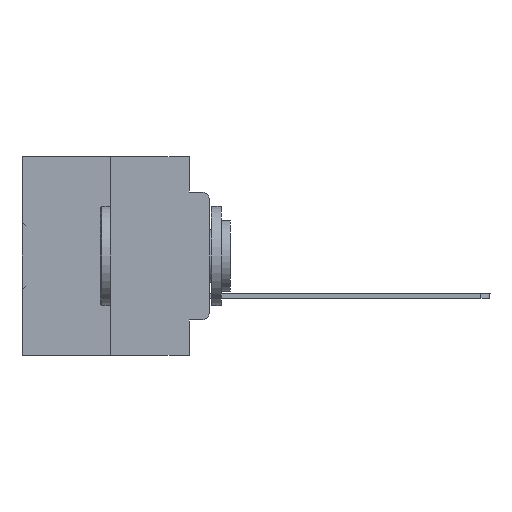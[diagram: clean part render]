
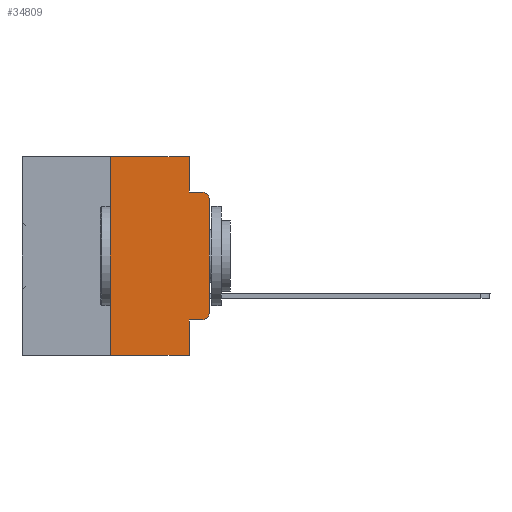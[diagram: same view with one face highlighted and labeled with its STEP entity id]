
A CAD part, left-side view. The second image highlights one B-rep face of the part: STEP entity #34809.
In plain terms, the highlighted planar face has unit normal (-1, 0, 0).
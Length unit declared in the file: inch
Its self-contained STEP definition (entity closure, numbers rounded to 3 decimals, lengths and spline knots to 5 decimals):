
#565 = VECTOR ( 'NONE', #27061, 39.37008 ) ;
#676 = CARTESIAN_POINT ( 'NONE',  ( 0., 0.051, -0.0885 ) ) ;
#716 = DIRECTION ( 'NONE',  ( -1., 0., 0. ) ) ;
#834 = CARTESIAN_POINT ( 'NONE',  ( 0., 0.051, -0.4115 ) ) ;
#895 = ORIENTED_EDGE ( 'NONE', *, *, #23090, .T. ) ;
#981 = LINE ( 'NONE', #23210, #13466 ) ;
#1661 = DIRECTION ( 'NONE',  ( 0., -1., 0. ) ) ;
#2982 = EDGE_CURVE ( 'NONE', #19522, #21882, #26167, .T. ) ;
#3348 = CARTESIAN_POINT ( 'NONE',  ( 0., 0.473, 0. ) ) ;
#4129 = CARTESIAN_POINT ( 'NONE',  ( 0., 0.473, -0.5 ) ) ;
#4515 = EDGE_CURVE ( 'NONE', #19522, #31676, #13533, .T. ) ;
#4795 = CARTESIAN_POINT ( 'NONE',  ( 0., 0., 0. ) ) ;
#4839 = VERTEX_POINT ( 'NONE', #7414 ) ;
#6192 = VECTOR ( 'NONE', #35903, 39.37008 ) ;
#6495 = EDGE_CURVE ( 'NONE', #4839, #33260, #25482, .T. ) ;
#6571 = ORIENTED_EDGE ( 'NONE', *, *, #23447, .T. ) ;
#7414 = CARTESIAN_POINT ( 'NONE',  ( 0., 0.25, -0.5 ) ) ;
#7558 = LINE ( 'NONE', #18197, #15893 ) ;
#7573 = VECTOR ( 'NONE', #21011, 39.37008 ) ;
#9270 = EDGE_CURVE ( 'NONE', #21882, #29329, #12738, .T. ) ;
#9669 = CARTESIAN_POINT ( 'NONE',  ( 0., 0., -0.3915 ) ) ;
#10078 = VECTOR ( 'NONE', #34612, 39.37008 ) ;
#10139 = LINE ( 'NONE', #4795, #32683 ) ;
#10311 = EDGE_LOOP ( 'NONE', ( #6571, #895, #25786, #10936, #17697, #33186, #24774, #27857, #26326, #21226 ) ) ;
#10936 = ORIENTED_EDGE ( 'NONE', *, *, #33438, .F. ) ;
#11402 = EDGE_CURVE ( 'NONE', #16914, #16169, #12222, .T. ) ;
#12222 = LINE ( 'NONE', #18078, #7573 ) ;
#12738 = CIRCLE ( 'NONE', #29735, 0.02 ) ;
#13162 = CARTESIAN_POINT ( 'NONE',  ( 0., 0.051, -0.4115 ) ) ;
#13466 = VECTOR ( 'NONE', #25590, 39.37008 ) ;
#13533 = LINE ( 'NONE', #24704, #6192 ) ;
#13666 = CARTESIAN_POINT ( 'NONE',  ( 0., 0.02, -0.1085 ) ) ;
#13837 = DIRECTION ( 'NONE',  ( 0., 0., -1. ) ) ;
#14575 = DIRECTION ( 'NONE',  ( 1., 0., 0. ) ) ;
#15657 = CARTESIAN_POINT ( 'NONE',  ( 0., 0.02, -0.0885 ) ) ;
#15854 = EDGE_CURVE ( 'NONE', #4839, #31676, #16072, .T. ) ;
#15893 = VECTOR ( 'NONE', #1661, 39.37008 ) ;
#16072 = LINE ( 'NONE', #4129, #565 ) ;
#16169 = VERTEX_POINT ( 'NONE', #15657 ) ;
#16354 = VECTOR ( 'NONE', #28792, 39.37008 ) ;
#16914 = VERTEX_POINT ( 'NONE', #676 ) ;
#17449 = AXIS2_PLACEMENT_3D ( 'NONE', #13666, #22075, #13837 ) ;
#17697 = ORIENTED_EDGE ( 'NONE', *, *, #28563, .F. ) ;
#18078 = CARTESIAN_POINT ( 'NONE',  ( 0., 0.051, -0.0885 ) ) ;
#18197 = CARTESIAN_POINT ( 'NONE',  ( 0., 0.473, 0. ) ) ;
#18350 = CARTESIAN_POINT ( 'NONE',  ( 0., 0.02, -0.3915 ) ) ;
#18533 = CARTESIAN_POINT ( 'NONE',  ( 0., 0., -0.1085 ) ) ;
#19384 = CARTESIAN_POINT ( 'NONE',  ( 0., 0.25, 0. ) ) ;
#19522 = VERTEX_POINT ( 'NONE', #13162 ) ;
#20610 = DIRECTION ( 'NONE',  ( 0., 0., -1. ) ) ;
#21011 = DIRECTION ( 'NONE',  ( 0., -1., 0. ) ) ;
#21090 = CARTESIAN_POINT ( 'NONE',  ( 0., 0.02, -0.4115 ) ) ;
#21226 = ORIENTED_EDGE ( 'NONE', *, *, #9270, .T. ) ;
#21882 = VERTEX_POINT ( 'NONE', #21090 ) ;
#22075 = DIRECTION ( 'NONE',  ( -1., 0., 0. ) ) ;
#22351 = CARTESIAN_POINT ( 'NONE',  ( 0., 0.051, -0.5 ) ) ;
#23090 = EDGE_CURVE ( 'NONE', #35263, #16169, #33846, .T. ) ;
#23126 = DIRECTION ( 'NONE',  ( 0., 0., -1. ) ) ;
#23210 = CARTESIAN_POINT ( 'NONE',  ( 0., 0.051, 0. ) ) ;
#23447 = EDGE_CURVE ( 'NONE', #29329, #35263, #10139, .T. ) ;
#24704 = CARTESIAN_POINT ( 'NONE',  ( 0., 0.051, 0. ) ) ;
#24774 = ORIENTED_EDGE ( 'NONE', *, *, #15854, .T. ) ;
#25482 = LINE ( 'NONE', #25670, #16354 ) ;
#25590 = DIRECTION ( 'NONE',  ( 0., 0., -1. ) ) ;
#25670 = CARTESIAN_POINT ( 'NONE',  ( 0., 0.25, 0. ) ) ;
#25786 = ORIENTED_EDGE ( 'NONE', *, *, #11402, .F. ) ;
#26167 = LINE ( 'NONE', #834, #10078 ) ;
#26326 = ORIENTED_EDGE ( 'NONE', *, *, #2982, .T. ) ;
#27061 = DIRECTION ( 'NONE',  ( 0., -1., 0. ) ) ;
#27185 = DIRECTION ( 'NONE',  ( 0., 0., 1. ) ) ;
#27857 = ORIENTED_EDGE ( 'NONE', *, *, #4515, .F. ) ;
#28486 = PLANE ( 'NONE',  #31221 ) ;
#28563 = EDGE_CURVE ( 'NONE', #33260, #34834, #7558, .T. ) ;
#28792 = DIRECTION ( 'NONE',  ( 0., 0., 1. ) ) ;
#29329 = VERTEX_POINT ( 'NONE', #9669 ) ;
#29593 = CARTESIAN_POINT ( 'NONE',  ( 0., 0.051, 0. ) ) ;
#29735 = AXIS2_PLACEMENT_3D ( 'NONE', #18350, #716, #23126 ) ;
#31221 = AXIS2_PLACEMENT_3D ( 'NONE', #3348, #14575, #20610 ) ;
#31251 = FACE_OUTER_BOUND ( 'NONE', #10311, .T. ) ;
#31676 = VERTEX_POINT ( 'NONE', #22351 ) ;
#32683 = VECTOR ( 'NONE', #27185, 39.37008 ) ;
#33186 = ORIENTED_EDGE ( 'NONE', *, *, #6495, .F. ) ;
#33260 = VERTEX_POINT ( 'NONE', #19384 ) ;
#33438 = EDGE_CURVE ( 'NONE', #34834, #16914, #981, .T. ) ;
#33846 = CIRCLE ( 'NONE', #17449, 0.02 ) ;
#34612 = DIRECTION ( 'NONE',  ( 0., -1., 0. ) ) ;
#34809 = ADVANCED_FACE ( 'NONE', ( #31251 ), #28486, .F. ) ;
#34834 = VERTEX_POINT ( 'NONE', #29593 ) ;
#35263 = VERTEX_POINT ( 'NONE', #18533 ) ;
#35903 = DIRECTION ( 'NONE',  ( 0., 0., -1. ) ) ;
